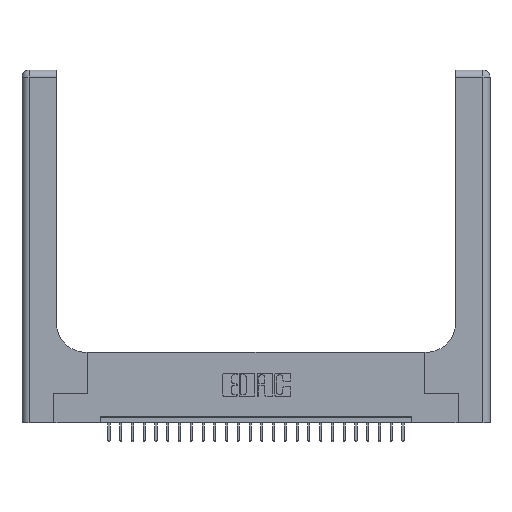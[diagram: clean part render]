
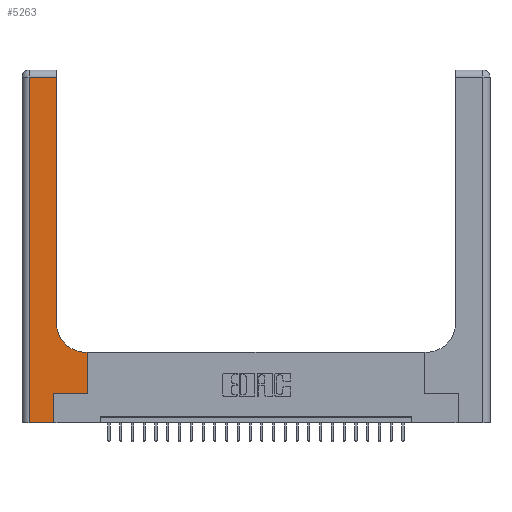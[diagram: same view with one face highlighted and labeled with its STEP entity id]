
A CAD part, top view. The second image highlights one B-rep face of the part: STEP entity #5263.
In plain terms, the highlighted planar face has unit normal (0, 0, 1).
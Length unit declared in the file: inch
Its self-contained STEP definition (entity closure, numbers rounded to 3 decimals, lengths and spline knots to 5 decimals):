
#233 = CARTESIAN_POINT ( 'NONE',  ( 0., 3., 0.37 ) ) ;
#496 = VERTEX_POINT ( 'NONE', #23182 ) ;
#503 = CARTESIAN_POINT ( 'NONE',  ( 0.06, 2.94, 0.37 ) ) ;
#760 = DIRECTION ( 'NONE',  ( 0., 1., 0. ) ) ;
#1598 = EDGE_CURVE ( 'NONE', #8297, #496, #21379, .T. ) ;
#2084 = CARTESIAN_POINT ( 'NONE',  ( 0.5415, 0.85, 0.37 ) ) ;
#2181 = VECTOR ( 'NONE', #5440, 39.37008 ) ;
#2270 = ORIENTED_EDGE ( 'NONE', *, *, #24662, .T. ) ;
#2616 = VERTEX_POINT ( 'NONE', #8769 ) ;
#2628 = DIRECTION ( 'NONE',  ( -1., 0., 0. ) ) ;
#3222 = VERTEX_POINT ( 'NONE', #14210 ) ;
#3409 = ORIENTED_EDGE ( 'NONE', *, *, #22604, .T. ) ;
#3441 = VECTOR ( 'NONE', #760, 39.37008 ) ;
#3968 = LINE ( 'NONE', #13544, #20591 ) ;
#4427 = DIRECTION ( 'NONE',  ( 0., 0., -1. ) ) ;
#5205 = CARTESIAN_POINT ( 'NONE',  ( 0.2915, 3., 0.37 ) ) ;
#5263 = ADVANCED_FACE ( 'NONE', ( #9531 ), #15024, .F. ) ;
#5303 = CARTESIAN_POINT ( 'NONE',  ( 0.06, 3., 0.37 ) ) ;
#5440 = DIRECTION ( 'NONE',  ( 0., 1., 0. ) ) ;
#5445 = VERTEX_POINT ( 'NONE', #23380 ) ;
#5558 = CARTESIAN_POINT ( 'NONE',  ( 0.06, 0., 0.37 ) ) ;
#5698 = CARTESIAN_POINT ( 'NONE',  ( 0.5585, 0.25, 0.37 ) ) ;
#5966 = LINE ( 'NONE', #5698, #19920 ) ;
#6271 = DIRECTION ( 'NONE',  ( 1., 0., 0. ) ) ;
#7272 = AXIS2_PLACEMENT_3D ( 'NONE', #2084, #24982, #22953 ) ;
#7525 = VECTOR ( 'NONE', #8427, 39.37008 ) ;
#8040 = LINE ( 'NONE', #5205, #3441 ) ;
#8297 = VERTEX_POINT ( 'NONE', #20640 ) ;
#8427 = DIRECTION ( 'NONE',  ( -1., 0., 0. ) ) ;
#8769 = CARTESIAN_POINT ( 'NONE',  ( 0.269, 0., 0.37 ) ) ;
#9125 = VERTEX_POINT ( 'NONE', #22268 ) ;
#9200 = EDGE_CURVE ( 'NONE', #3222, #5445, #25255, .T. ) ;
#9531 = FACE_OUTER_BOUND ( 'NONE', #9539, .T. ) ;
#9539 = EDGE_LOOP ( 'NONE', ( #2270, #22573, #18615, #3409, #24358, #25441, #25001, #16121, #16486 ) ) ;
#9891 = DIRECTION ( 'NONE',  ( 0., 1., 0. ) ) ;
#10002 = LINE ( 'NONE', #11722, #2181 ) ;
#10410 = EDGE_CURVE ( 'NONE', #9125, #8297, #3968, .T. ) ;
#10526 = EDGE_CURVE ( 'NONE', #2616, #3222, #10002, .T. ) ;
#10984 = LINE ( 'NONE', #5303, #24012 ) ;
#11043 = VECTOR ( 'NONE', #6271, 39.37008 ) ;
#11270 = DIRECTION ( 'NONE',  ( -1., 0., 0. ) ) ;
#11722 = CARTESIAN_POINT ( 'NONE',  ( 0.269, 0., 0.37 ) ) ;
#12380 = CARTESIAN_POINT ( 'NONE',  ( 0.269, 0.25, 0.37 ) ) ;
#12399 = LINE ( 'NONE', #22774, #7525 ) ;
#13544 = CARTESIAN_POINT ( 'NONE',  ( 0.2915, 0.6, 0.37 ) ) ;
#13724 = VERTEX_POINT ( 'NONE', #503 ) ;
#14210 = CARTESIAN_POINT ( 'NONE',  ( 0.269, 0.25, 0.37 ) ) ;
#14282 = DIRECTION ( 'NONE',  ( 1., 0., 0. ) ) ;
#15024 = PLANE ( 'NONE',  #17578 ) ;
#15559 = LINE ( 'NONE', #18881, #11043 ) ;
#15646 = EDGE_CURVE ( 'NONE', #19246, #13724, #12399, .T. ) ;
#16121 = ORIENTED_EDGE ( 'NONE', *, *, #10410, .T. ) ;
#16486 = ORIENTED_EDGE ( 'NONE', *, *, #1598, .T. ) ;
#17578 = AXIS2_PLACEMENT_3D ( 'NONE', #233, #4427, #2628 ) ;
#17727 = EDGE_CURVE ( 'NONE', #13724, #18785, #10984, .T. ) ;
#17914 = DIRECTION ( 'NONE',  ( 0., -1., 0. ) ) ;
#18615 = ORIENTED_EDGE ( 'NONE', *, *, #17727, .T. ) ;
#18785 = VERTEX_POINT ( 'NONE', #5558 ) ;
#18881 = CARTESIAN_POINT ( 'NONE',  ( 0., 0., 0.37 ) ) ;
#19246 = VERTEX_POINT ( 'NONE', #23915 ) ;
#19920 = VECTOR ( 'NONE', #9891, 39.37008 ) ;
#20591 = VECTOR ( 'NONE', #11270, 39.37008 ) ;
#20640 = CARTESIAN_POINT ( 'NONE',  ( 0.5415, 0.6, 0.37 ) ) ;
#21379 = CIRCLE ( 'NONE', #7272, 0.25 ) ;
#22268 = CARTESIAN_POINT ( 'NONE',  ( 0.5585, 0.6, 0.37 ) ) ;
#22573 = ORIENTED_EDGE ( 'NONE', *, *, #15646, .T. ) ;
#22604 = EDGE_CURVE ( 'NONE', #18785, #2616, #15559, .T. ) ;
#22774 = CARTESIAN_POINT ( 'NONE',  ( 0., 2.94, 0.37 ) ) ;
#22953 = DIRECTION ( 'NONE',  ( 1., 0., 0. ) ) ;
#23182 = CARTESIAN_POINT ( 'NONE',  ( 0.2915, 0.85, 0.37 ) ) ;
#23277 = VECTOR ( 'NONE', #14282, 39.37008 ) ;
#23380 = CARTESIAN_POINT ( 'NONE',  ( 0.5585, 0.25, 0.37 ) ) ;
#23915 = CARTESIAN_POINT ( 'NONE',  ( 0.2915, 2.94, 0.37 ) ) ;
#24012 = VECTOR ( 'NONE', #17914, 39.37008 ) ;
#24358 = ORIENTED_EDGE ( 'NONE', *, *, #10526, .T. ) ;
#24662 = EDGE_CURVE ( 'NONE', #496, #19246, #8040, .T. ) ;
#24982 = DIRECTION ( 'NONE',  ( 0., 0., -1. ) ) ;
#25001 = ORIENTED_EDGE ( 'NONE', *, *, #26720, .T. ) ;
#25255 = LINE ( 'NONE', #12380, #23277 ) ;
#25441 = ORIENTED_EDGE ( 'NONE', *, *, #9200, .T. ) ;
#26720 = EDGE_CURVE ( 'NONE', #5445, #9125, #5966, .T. ) ;
